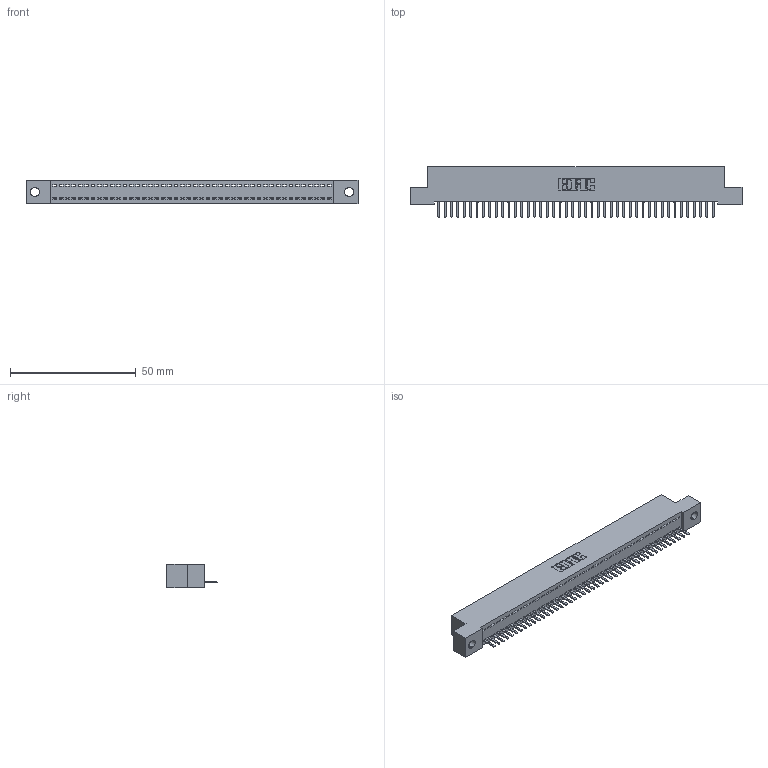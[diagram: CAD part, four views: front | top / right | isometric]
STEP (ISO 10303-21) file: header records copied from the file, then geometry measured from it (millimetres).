
FILE_DESCRIPTION (( 'STEP AP203' ), '1' );
FILE_NAME ('342-044-520-102.STEP', '2018-08-12T14:12:25', ( '' ), ( '' ), 'SwSTEP 2.0', 'SolidWorks 2016', '' );
FILE_SCHEMA (( 'CONFIG_CONTROL_DESIGN' ));
Length unit declared in the file: inch
Products named in the file (3): 345-292-001_345-293-120; 342-044-520-102; 342 Part_.128 Slot
Assembly tree (45 placements, depth 2):
  342-044-520-102
    342 Part_.128 Slot
    345-292-001_345-293-120  x44
Bounding box: 132.08 x 20.02 x 9.4 mm (x, y, z)
Volume: 11409.4 mm3; surface area: 16146.4 mm2
Topology: 45 solids, 45 shells, 2842 faces, 8407 edges, 5486 vertices
Faces by surface type: plane 2006, cylinder 836
Entity records: 26757 total; most frequent: CARTESIAN_POINT 4634, ORIENTED_EDGE 4602, DIRECTION 3893, EDGE_CURVE 2301, LINE 2169, VECTOR 2169, VERTEX_POINT 1530, AXIS2_PLACEMENT_3D 862
